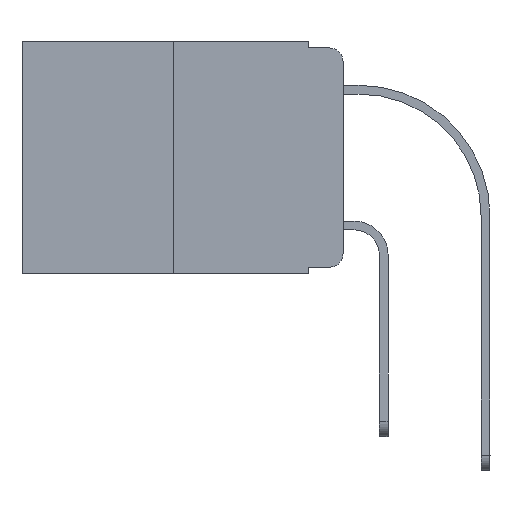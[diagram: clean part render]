
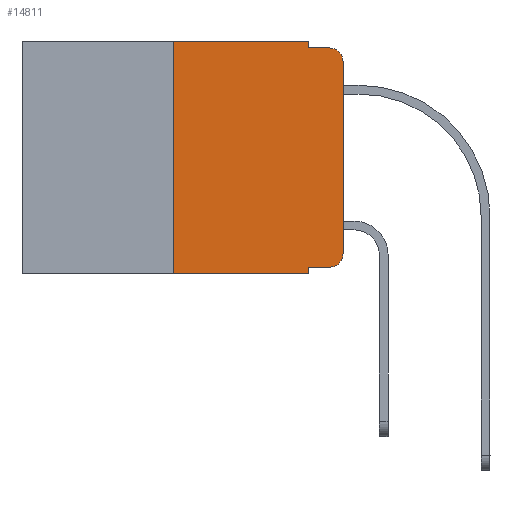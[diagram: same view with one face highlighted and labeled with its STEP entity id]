
A CAD part, left-side view. The second image highlights one B-rep face of the part: STEP entity #14811.
In plain terms, the highlighted planar face has unit normal (-1, 0, 0).
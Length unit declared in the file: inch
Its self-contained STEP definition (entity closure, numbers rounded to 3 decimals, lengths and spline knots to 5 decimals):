
#471 = VECTOR ( 'NONE', #5413, 39.37008 ) ;
#637 = EDGE_CURVE ( 'NONE', #5728, #10363, #3262, .T. ) ;
#642 = DIRECTION ( 'NONE',  ( -1., 0., 0. ) ) ;
#1151 = DIRECTION ( 'NONE',  ( 0., 0., -1. ) ) ;
#1235 = CARTESIAN_POINT ( 'NONE',  ( 0., 0.051, -0.343 ) ) ;
#1263 = EDGE_CURVE ( 'NONE', #5418, #5728, #13044, .T. ) ;
#1296 = FACE_OUTER_BOUND ( 'NONE', #2205, .T. ) ;
#1528 = ORIENTED_EDGE ( 'NONE', *, *, #1263, .T. ) ;
#1721 = CIRCLE ( 'NONE', #2005, 0.02 ) ;
#2005 = AXIS2_PLACEMENT_3D ( 'NONE', #14641, #642, #1151 ) ;
#2205 = EDGE_LOOP ( 'NONE', ( #1528, #5017, #7956, #5227, #15507, #15278, #14796, #14761, #13613, #10044 ) ) ;
#2288 = VERTEX_POINT ( 'NONE', #2431 ) ;
#2431 = CARTESIAN_POINT ( 'NONE',  ( 0., 0.051, 0. ) ) ;
#2628 = EDGE_CURVE ( 'NONE', #10229, #10363, #17701, .T. ) ;
#2684 = DIRECTION ( 'NONE',  ( 0., -1., 0. ) ) ;
#3009 = CARTESIAN_POINT ( 'NONE',  ( 0., 0.473, -0.343 ) ) ;
#3098 = VERTEX_POINT ( 'NONE', #6428 ) ;
#3119 = EDGE_CURVE ( 'NONE', #7321, #2288, #15561, .T. ) ;
#3176 = VECTOR ( 'NONE', #13238, 39.37008 ) ;
#3262 = CIRCLE ( 'NONE', #15804, 0.02 ) ;
#3333 = CARTESIAN_POINT ( 'NONE',  ( 0., 0.25, 0. ) ) ;
#3653 = CARTESIAN_POINT ( 'NONE',  ( 0., 0.02, -0.01 ) ) ;
#4259 = EDGE_CURVE ( 'NONE', #2288, #10229, #13074, .T. ) ;
#4375 = CARTESIAN_POINT ( 'NONE',  ( 0., 0., -0.313 ) ) ;
#5016 = LINE ( 'NONE', #16240, #16598 ) ;
#5017 = ORIENTED_EDGE ( 'NONE', *, *, #637, .T. ) ;
#5227 = ORIENTED_EDGE ( 'NONE', *, *, #4259, .F. ) ;
#5360 = DIRECTION ( 'NONE',  ( 1., 0., 0. ) ) ;
#5413 = DIRECTION ( 'NONE',  ( 0., 0., -1. ) ) ;
#5418 = VERTEX_POINT ( 'NONE', #4375 ) ;
#5545 = PLANE ( 'NONE',  #6173 ) ;
#5623 = CARTESIAN_POINT ( 'NONE',  ( 0., 0.051, -0.01 ) ) ;
#5728 = VERTEX_POINT ( 'NONE', #16578 ) ;
#6173 = AXIS2_PLACEMENT_3D ( 'NONE', #12359, #5360, #7092 ) ;
#6252 = CARTESIAN_POINT ( 'NONE',  ( 0., 0.051, 0. ) ) ;
#6428 = CARTESIAN_POINT ( 'NONE',  ( 0., 0.02, -0.333 ) ) ;
#7092 = DIRECTION ( 'NONE',  ( 0., 0., -1. ) ) ;
#7245 = VECTOR ( 'NONE', #8568, 39.37008 ) ;
#7321 = VERTEX_POINT ( 'NONE', #3333 ) ;
#7516 = EDGE_CURVE ( 'NONE', #3098, #5418, #1721, .T. ) ;
#7956 = ORIENTED_EDGE ( 'NONE', *, *, #2628, .F. ) ;
#8135 = VECTOR ( 'NONE', #12513, 39.37008 ) ;
#8475 = LINE ( 'NONE', #3009, #7245 ) ;
#8487 = VECTOR ( 'NONE', #10246, 39.37008 ) ;
#8568 = DIRECTION ( 'NONE',  ( 0., -1., 0. ) ) ;
#9392 = EDGE_CURVE ( 'NONE', #17148, #17346, #17957, .T. ) ;
#10044 = ORIENTED_EDGE ( 'NONE', *, *, #7516, .T. ) ;
#10229 = VERTEX_POINT ( 'NONE', #5623 ) ;
#10246 = DIRECTION ( 'NONE',  ( 0., 0., -1. ) ) ;
#10363 = VERTEX_POINT ( 'NONE', #3653 ) ;
#10434 = VECTOR ( 'NONE', #2684, 39.37008 ) ;
#10466 = CARTESIAN_POINT ( 'NONE',  ( 0., 0.051, -0.333 ) ) ;
#10473 = EDGE_CURVE ( 'NONE', #17148, #3098, #10488, .T. ) ;
#10488 = LINE ( 'NONE', #16108, #3176 ) ;
#11152 = EDGE_CURVE ( 'NONE', #14552, #17346, #8475, .T. ) ;
#11337 = EDGE_CURVE ( 'NONE', #14552, #7321, #5016, .T. ) ;
#11814 = DIRECTION ( 'NONE',  ( 0., 0., 1. ) ) ;
#12359 = CARTESIAN_POINT ( 'NONE',  ( 0., 0.473, 0. ) ) ;
#12419 = CARTESIAN_POINT ( 'NONE',  ( 0., 0.473, 0. ) ) ;
#12513 = DIRECTION ( 'NONE',  ( 0., -1., 0. ) ) ;
#12714 = CARTESIAN_POINT ( 'NONE',  ( 0., 0.02, -0.03 ) ) ;
#12801 = DIRECTION ( 'NONE',  ( 0., 0., -1. ) ) ;
#13044 = LINE ( 'NONE', #14704, #17039 ) ;
#13074 = LINE ( 'NONE', #6252, #8487 ) ;
#13238 = DIRECTION ( 'NONE',  ( 0., -1., 0. ) ) ;
#13613 = ORIENTED_EDGE ( 'NONE', *, *, #10473, .T. ) ;
#14552 = VERTEX_POINT ( 'NONE', #16053 ) ;
#14641 = CARTESIAN_POINT ( 'NONE',  ( 0., 0.02, -0.313 ) ) ;
#14704 = CARTESIAN_POINT ( 'NONE',  ( 0., 0., 0. ) ) ;
#14761 = ORIENTED_EDGE ( 'NONE', *, *, #9392, .F. ) ;
#14796 = ORIENTED_EDGE ( 'NONE', *, *, #11152, .T. ) ;
#14811 = ADVANCED_FACE ( 'NONE', ( #1296 ), #5545, .F. ) ;
#15079 = CARTESIAN_POINT ( 'NONE',  ( 0., 0.051, 0. ) ) ;
#15213 = CARTESIAN_POINT ( 'NONE',  ( 0., 0.051, -0.01 ) ) ;
#15278 = ORIENTED_EDGE ( 'NONE', *, *, #11337, .F. ) ;
#15507 = ORIENTED_EDGE ( 'NONE', *, *, #3119, .F. ) ;
#15561 = LINE ( 'NONE', #12419, #8135 ) ;
#15673 = DIRECTION ( 'NONE',  ( -1., 0., 0. ) ) ;
#15804 = AXIS2_PLACEMENT_3D ( 'NONE', #12714, #15673, #12801 ) ;
#16053 = CARTESIAN_POINT ( 'NONE',  ( 0., 0.25, -0.343 ) ) ;
#16108 = CARTESIAN_POINT ( 'NONE',  ( 0., 0.051, -0.333 ) ) ;
#16240 = CARTESIAN_POINT ( 'NONE',  ( 0., 0.25, 0. ) ) ;
#16578 = CARTESIAN_POINT ( 'NONE',  ( 0., 0., -0.03 ) ) ;
#16598 = VECTOR ( 'NONE', #11814, 39.37008 ) ;
#17039 = VECTOR ( 'NONE', #17311, 39.37008 ) ;
#17148 = VERTEX_POINT ( 'NONE', #10466 ) ;
#17311 = DIRECTION ( 'NONE',  ( 0., 0., 1. ) ) ;
#17346 = VERTEX_POINT ( 'NONE', #1235 ) ;
#17701 = LINE ( 'NONE', #15213, #10434 ) ;
#17957 = LINE ( 'NONE', #15079, #471 ) ;
